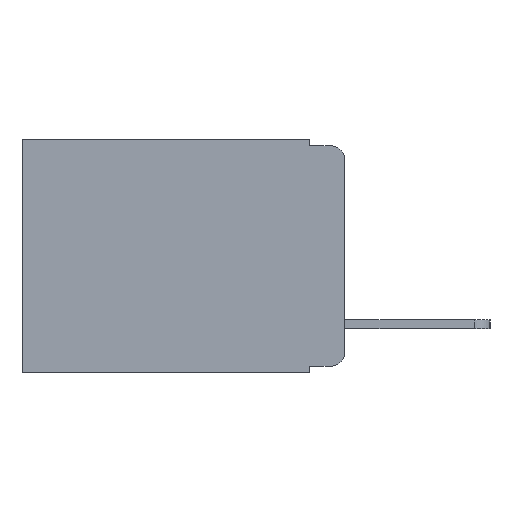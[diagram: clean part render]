
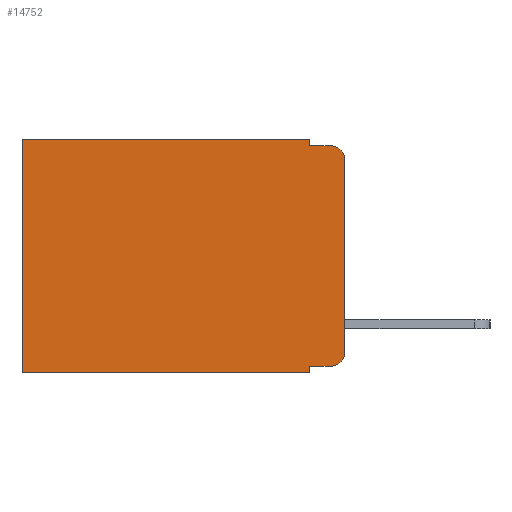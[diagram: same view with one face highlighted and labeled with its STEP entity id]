
A CAD part, left-side view. The second image highlights one B-rep face of the part: STEP entity #14752.
In plain terms, the highlighted planar face has unit normal (-1, 0, 0).
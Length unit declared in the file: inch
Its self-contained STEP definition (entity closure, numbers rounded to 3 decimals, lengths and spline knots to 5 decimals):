
#113 = CARTESIAN_POINT ( 'NONE',  ( 0.298, 0., -0.313 ) ) ;
#392 = DIRECTION ( 'NONE',  ( 0., -1., 0. ) ) ;
#448 = ORIENTED_EDGE ( 'NONE', *, *, #12778, .T. ) ;
#484 = LINE ( 'NONE', #4899, #11077 ) ;
#741 = AXIS2_PLACEMENT_3D ( 'NONE', #16867, #16671, #16656 ) ;
#760 = VERTEX_POINT ( 'NONE', #11796 ) ;
#767 = EDGE_CURVE ( 'NONE', #4199, #760, #2318, .T. ) ;
#1073 = CARTESIAN_POINT ( 'NONE',  ( 0.298, 0.051, -0.333 ) ) ;
#1808 = EDGE_CURVE ( 'NONE', #4199, #11326, #8332, .T. ) ;
#1837 = EDGE_CURVE ( 'NONE', #2020, #4052, #484, .T. ) ;
#1929 = LINE ( 'NONE', #3195, #16128 ) ;
#2020 = VERTEX_POINT ( 'NONE', #1073 ) ;
#2165 = ORIENTED_EDGE ( 'NONE', *, *, #16563, .T. ) ;
#2318 = CIRCLE ( 'NONE', #741, 0.02 ) ;
#3194 = DIRECTION ( 'NONE',  ( 0., 1., 0. ) ) ;
#3195 = CARTESIAN_POINT ( 'NONE',  ( 0.298, 0.051, -0.01 ) ) ;
#3373 = VECTOR ( 'NONE', #17464, 39.37008 ) ;
#3512 = LINE ( 'NONE', #17643, #17214 ) ;
#3793 = EDGE_CURVE ( 'NONE', #6362, #11326, #17016, .T. ) ;
#3830 = PLANE ( 'NONE',  #10051 ) ;
#4052 = VERTEX_POINT ( 'NONE', #6993 ) ;
#4199 = VERTEX_POINT ( 'NONE', #17442 ) ;
#4442 = DIRECTION ( 'NONE',  ( 0., 0., -1. ) ) ;
#4702 = VECTOR ( 'NONE', #4442, 39.37008 ) ;
#4899 = CARTESIAN_POINT ( 'NONE',  ( 0.298, 0.051, 0. ) ) ;
#5241 = CARTESIAN_POINT ( 'NONE',  ( 0.298, 0., 0. ) ) ;
#5906 = VECTOR ( 'NONE', #11560, 39.37008 ) ;
#5999 = ORIENTED_EDGE ( 'NONE', *, *, #6120, .F. ) ;
#6039 = VECTOR ( 'NONE', #13687, 39.37008 ) ;
#6120 = EDGE_CURVE ( 'NONE', #15396, #760, #1929, .T. ) ;
#6362 = VERTEX_POINT ( 'NONE', #14677 ) ;
#6658 = ORIENTED_EDGE ( 'NONE', *, *, #767, .T. ) ;
#6667 = DIRECTION ( 'NONE',  ( 0., 0., -1. ) ) ;
#6805 = EDGE_CURVE ( 'NONE', #10639, #9428, #9442, .T. ) ;
#6993 = CARTESIAN_POINT ( 'NONE',  ( 0.298, 0.051, -0.343 ) ) ;
#7098 = LINE ( 'NONE', #16104, #3373 ) ;
#8014 = CARTESIAN_POINT ( 'NONE',  ( 0.298, 0.02, -0.313 ) ) ;
#8296 = ORIENTED_EDGE ( 'NONE', *, *, #6805, .T. ) ;
#8332 = LINE ( 'NONE', #9390, #4702 ) ;
#8431 = DIRECTION ( 'NONE',  ( 0., 0., -1. ) ) ;
#8508 = ORIENTED_EDGE ( 'NONE', *, *, #1808, .F. ) ;
#8925 = FACE_OUTER_BOUND ( 'NONE', #12010, .T. ) ;
#9324 = LINE ( 'NONE', #9997, #16187 ) ;
#9390 = CARTESIAN_POINT ( 'NONE',  ( 0.298, 0., 0. ) ) ;
#9428 = VERTEX_POINT ( 'NONE', #11147 ) ;
#9442 = LINE ( 'NONE', #17012, #5906 ) ;
#9478 = CARTESIAN_POINT ( 'NONE',  ( 0.298, 0.473, 0. ) ) ;
#9997 = CARTESIAN_POINT ( 'NONE',  ( 0.298, 0., 0. ) ) ;
#10016 = EDGE_CURVE ( 'NONE', #17362, #15396, #16875, .T. ) ;
#10051 = AXIS2_PLACEMENT_3D ( 'NONE', #5241, #14760, #6667 ) ;
#10618 = ORIENTED_EDGE ( 'NONE', *, *, #11743, .F. ) ;
#10639 = VERTEX_POINT ( 'NONE', #9478 ) ;
#10775 = ORIENTED_EDGE ( 'NONE', *, *, #3793, .T. ) ;
#10824 = DIRECTION ( 'NONE',  ( 0., -1., 0. ) ) ;
#11045 = ORIENTED_EDGE ( 'NONE', *, *, #1837, .F. ) ;
#11077 = VECTOR ( 'NONE', #16826, 39.37008 ) ;
#11147 = CARTESIAN_POINT ( 'NONE',  ( 0.298, 0.473, -0.343 ) ) ;
#11326 = VERTEX_POINT ( 'NONE', #113 ) ;
#11344 = CARTESIAN_POINT ( 'NONE',  ( 0.298, 0.051, 0. ) ) ;
#11560 = DIRECTION ( 'NONE',  ( 0., 0., -1. ) ) ;
#11743 = EDGE_CURVE ( 'NONE', #4052, #9428, #7098, .T. ) ;
#11796 = CARTESIAN_POINT ( 'NONE',  ( 0.298, 0.02, -0.01 ) ) ;
#12010 = EDGE_LOOP ( 'NONE', ( #8508, #6658, #5999, #12748, #448, #8296, #10618, #11045, #2165, #10775 ) ) ;
#12320 = CARTESIAN_POINT ( 'NONE',  ( 0.298, 0.051, 0. ) ) ;
#12748 = ORIENTED_EDGE ( 'NONE', *, *, #10016, .F. ) ;
#12778 = EDGE_CURVE ( 'NONE', #17362, #10639, #9324, .T. ) ;
#13687 = DIRECTION ( 'NONE',  ( 0., 0., -1. ) ) ;
#14677 = CARTESIAN_POINT ( 'NONE',  ( 0.298, 0.02, -0.333 ) ) ;
#14752 = ADVANCED_FACE ( 'NONE', ( #8925 ), #3830, .F. ) ;
#14760 = DIRECTION ( 'NONE',  ( 1., 0., 0. ) ) ;
#15396 = VERTEX_POINT ( 'NONE', #17191 ) ;
#16104 = CARTESIAN_POINT ( 'NONE',  ( 0.298, 0., -0.343 ) ) ;
#16128 = VECTOR ( 'NONE', #392, 39.37008 ) ;
#16187 = VECTOR ( 'NONE', #3194, 39.37008 ) ;
#16563 = EDGE_CURVE ( 'NONE', #2020, #6362, #3512, .T. ) ;
#16656 = DIRECTION ( 'NONE',  ( 0., 0., -1. ) ) ;
#16671 = DIRECTION ( 'NONE',  ( -1., 0., 0. ) ) ;
#16826 = DIRECTION ( 'NONE',  ( 0., 0., -1. ) ) ;
#16867 = CARTESIAN_POINT ( 'NONE',  ( 0.298, 0.02, -0.03 ) ) ;
#16875 = LINE ( 'NONE', #12320, #6039 ) ;
#17012 = CARTESIAN_POINT ( 'NONE',  ( 0.298, 0.473, 0. ) ) ;
#17016 = CIRCLE ( 'NONE', #17156, 0.02 ) ;
#17156 = AXIS2_PLACEMENT_3D ( 'NONE', #8014, #17507, #8431 ) ;
#17191 = CARTESIAN_POINT ( 'NONE',  ( 0.298, 0.051, -0.01 ) ) ;
#17214 = VECTOR ( 'NONE', #10824, 39.37008 ) ;
#17362 = VERTEX_POINT ( 'NONE', #11344 ) ;
#17442 = CARTESIAN_POINT ( 'NONE',  ( 0.298, 0., -0.03 ) ) ;
#17464 = DIRECTION ( 'NONE',  ( 0., 1., 0. ) ) ;
#17507 = DIRECTION ( 'NONE',  ( -1., 0., 0. ) ) ;
#17643 = CARTESIAN_POINT ( 'NONE',  ( 0.298, 0.051, -0.333 ) ) ;
